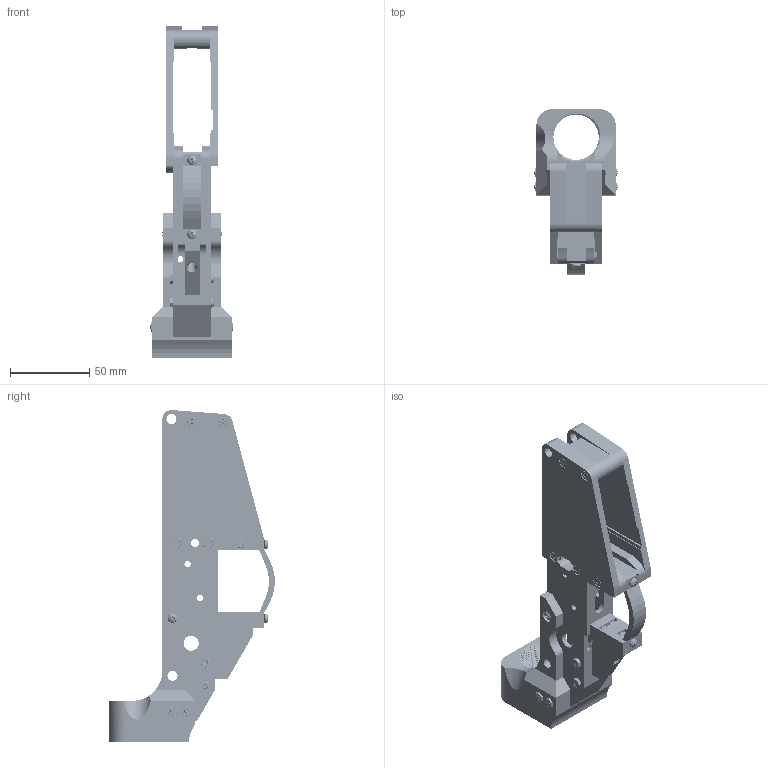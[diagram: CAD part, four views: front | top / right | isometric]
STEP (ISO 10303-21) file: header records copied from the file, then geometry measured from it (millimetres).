
FILE_DESCRIPTION (( 'STEP AP214' ), '1' );
FILE_NAME ('Reinforced_Assembly.step', '2015-06-12T16:51:56', ( '' ), ( '' ), 'SwSTEP 2.0', 'SolidWorks 2015', '' );
FILE_SCHEMA (( 'AUTOMOTIVE_DESIGN' ));
Length unit declared in the file: millimetre
Products named in the file (16): Reinforced_Assembly; M3_Nut_94150A325; M3_50mm_92000A139; M3_30mm_92000A132; M3_25mm_92000A130; M3_10mm_92000A120; Reinforced_Trigger_Guard; Reinforced_Mag_Well_Front; Reinforced_Mag_Well_Left; Reinforced_Mag_Well_Right; Reinforced_Mag_Well_Rear; Reinforced_Fire_Control_Well_Bottom; Reinforced_Grip_Part; Reinforced_Side_Left; Reinforced_Side_Right; Reinforced_Buffer
Assembly tree (40 placements, depth 2):
  Reinforced_Assembly
    Reinforced_Buffer
    Reinforced_Side_Right
    Reinforced_Side_Left
    Reinforced_Grip_Part
    Reinforced_Fire_Control_Well_Bottom
    Reinforced_Mag_Well_Rear
    Reinforced_Mag_Well_Right
    Reinforced_Mag_Well_Left
    Reinforced_Mag_Well_Front
    Reinforced_Trigger_Guard
    M3_10mm_92000A120  x6
    M3_25mm_92000A130  x2
    M3_30mm_92000A132  x5
    M3_50mm_92000A139  x2
    M3_Nut_94150A325  x15
Bounding box: 52.44 x 104.63 x 209.51 mm (x, y, z)
Volume: 177198.3 mm3; surface area: 95146.5 mm2
Topology: 40 solids, 40 shells, 5579 faces, 16059 edges, 10595 vertices
Faces by surface type: cylinder 4213, plane 746, cone 413, bspline 117, torus 60, sphere 30
Entity records: 124208 total; most frequent: CARTESIAN_POINT 77295, ORIENTED_EDGE 11670, DIRECTION 7871, EDGE_CURVE 5835, VERTEX_POINT 3872, AXIS2_PLACEMENT_3D 2730, VECTOR 2411, LINE 2411
